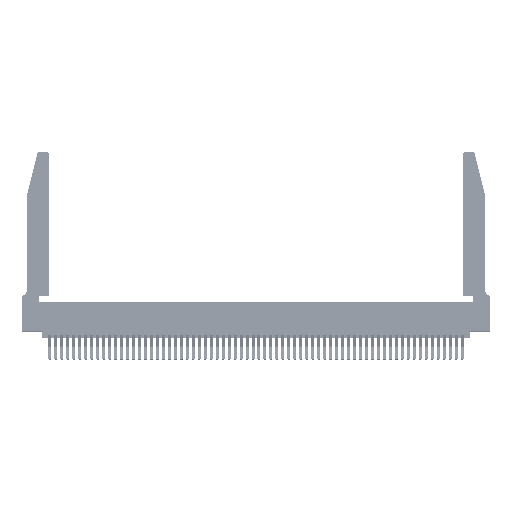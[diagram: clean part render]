
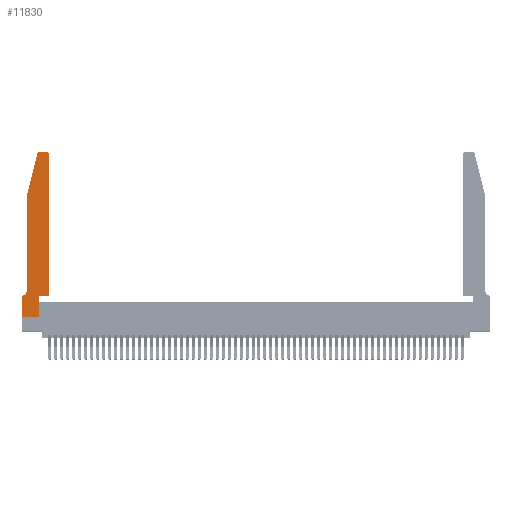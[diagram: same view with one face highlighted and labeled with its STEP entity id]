
A CAD part, top view. The second image highlights one B-rep face of the part: STEP entity #11830.
In plain terms, the highlighted planar face has unit normal (0, 0, 1).
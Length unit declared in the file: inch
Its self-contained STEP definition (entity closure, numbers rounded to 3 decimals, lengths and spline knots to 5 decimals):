
#631 = DIRECTION ( 'NONE',  ( 0., 0., 1. ) ) ;
#991 = LINE ( 'NONE', #21678, #45772 ) ;
#1443 = CARTESIAN_POINT ( 'NONE',  ( 0.4505, 0.35, 0.37 ) ) ;
#1514 = DIRECTION ( 'NONE',  ( 1., 0., 0. ) ) ;
#3117 = ORIENTED_EDGE ( 'NONE', *, *, #33888, .T. ) ;
#3269 = LINE ( 'NONE', #51267, #35183 ) ;
#3454 = CARTESIAN_POINT ( 'NONE',  ( 0.0755, 2., 0.37 ) ) ;
#3655 = VERTEX_POINT ( 'NONE', #53787 ) ;
#4149 = DIRECTION ( 'NONE',  ( 0., 0., 1. ) ) ;
#4368 = VERTEX_POINT ( 'NONE', #55041 ) ;
#4823 = VERTEX_POINT ( 'NONE', #53492 ) ;
#5504 = LINE ( 'NONE', #21820, #50225 ) ;
#7481 = CARTESIAN_POINT ( 'NONE',  ( 0.0055, 0.42, 0.37 ) ) ;
#7832 = DIRECTION ( 'NONE',  ( 0., -1., 0. ) ) ;
#9919 = ORIENTED_EDGE ( 'NONE', *, *, #21206, .T. ) ;
#10072 = EDGE_CURVE ( 'NONE', #13642, #23403, #991, .T. ) ;
#10275 = CARTESIAN_POINT ( 'NONE',  ( 0., 0., 0.37 ) ) ;
#10385 = VERTEX_POINT ( 'NONE', #10572 ) ;
#10572 = CARTESIAN_POINT ( 'NONE',  ( 0.284, 2.75, 0.37 ) ) ;
#10621 = CIRCLE ( 'NONE', #30736, 0.03 ) ;
#11830 = ADVANCED_FACE ( 'NONE', ( #29596 ), #52591, .T. ) ;
#11868 = DIRECTION ( 'NONE',  ( -1., 0., 0. ) ) ;
#13106 = ORIENTED_EDGE ( 'NONE', *, *, #21779, .T. ) ;
#13225 = DIRECTION ( 'NONE',  ( -1., 0., 0. ) ) ;
#13642 = VERTEX_POINT ( 'NONE', #27111 ) ;
#15131 = ORIENTED_EDGE ( 'NONE', *, *, #39594, .T. ) ;
#15133 = EDGE_CURVE ( 'NONE', #37219, #13642, #16375, .T. ) ;
#15163 = AXIS2_PLACEMENT_3D ( 'NONE', #22401, #631, #31086 ) ;
#15586 = EDGE_CURVE ( 'NONE', #3655, #22832, #49420, .T. ) ;
#16375 = CIRCLE ( 'NONE', #28686, 0.07 ) ;
#16689 = CARTESIAN_POINT ( 'NONE',  ( 0.4505, 0.35, 0.37 ) ) ;
#17494 = DIRECTION ( 'NONE',  ( -1., 0., 0. ) ) ;
#17820 = CARTESIAN_POINT ( 'NONE',  ( 0.4205, 2.75, 0.37 ) ) ;
#18159 = AXIS2_PLACEMENT_3D ( 'NONE', #30188, #4149, #34513 ) ;
#18362 = CARTESIAN_POINT ( 'NONE',  ( 0.25487, 2.72718, 0.37 ) ) ;
#18867 = ORIENTED_EDGE ( 'NONE', *, *, #54204, .T. ) ;
#18880 = VERTEX_POINT ( 'NONE', #17820 ) ;
#20620 = ORIENTED_EDGE ( 'NONE', *, *, #54653, .T. ) ;
#21063 = DIRECTION ( 'NONE',  ( 0., 1., 0. ) ) ;
#21206 = EDGE_CURVE ( 'NONE', #29919, #3655, #3269, .T. ) ;
#21678 = CARTESIAN_POINT ( 'NONE',  ( 0.0755, 0.35, 0.37 ) ) ;
#21779 = EDGE_CURVE ( 'NONE', #4823, #37219, #29715, .T. ) ;
#21820 = CARTESIAN_POINT ( 'NONE',  ( 0.2605, 2.75, 0.37 ) ) ;
#22352 = DIRECTION ( 'NONE',  ( 0., 0., 1. ) ) ;
#22401 = CARTESIAN_POINT ( 'NONE',  ( 0., 0.35, 0.37 ) ) ;
#22832 = VERTEX_POINT ( 'NONE', #1443 ) ;
#23403 = VERTEX_POINT ( 'NONE', #35562 ) ;
#24073 = CIRCLE ( 'NONE', #18159, 0.03 ) ;
#24998 = VERTEX_POINT ( 'NONE', #18362 ) ;
#27111 = CARTESIAN_POINT ( 'NONE',  ( 0.0055, 0.35, 0.37 ) ) ;
#27394 = LINE ( 'NONE', #41451, #50333 ) ;
#27542 = ORIENTED_EDGE ( 'NONE', *, *, #10072, .T. ) ;
#28374 = VECTOR ( 'NONE', #7832, 39.37008 ) ;
#28686 = AXIS2_PLACEMENT_3D ( 'NONE', #7481, #37790, #11868 ) ;
#29538 = ORIENTED_EDGE ( 'NONE', *, *, #15133, .T. ) ;
#29596 = FACE_OUTER_BOUND ( 'NONE', #49045, .T. ) ;
#29715 = LINE ( 'NONE', #3454, #28374 ) ;
#29919 = VERTEX_POINT ( 'NONE', #52624 ) ;
#30188 = CARTESIAN_POINT ( 'NONE',  ( 0.4205, 2.72, 0.37 ) ) ;
#30736 = AXIS2_PLACEMENT_3D ( 'NONE', #48177, #22352, #52539 ) ;
#31086 = DIRECTION ( 'NONE',  ( 1., 0., 0. ) ) ;
#33638 = ORIENTED_EDGE ( 'NONE', *, *, #54966, .T. ) ;
#33888 = EDGE_CURVE ( 'NONE', #22832, #54137, #46486, .T. ) ;
#34084 = LINE ( 'NONE', #34825, #55682 ) ;
#34489 = CARTESIAN_POINT ( 'NONE',  ( 0.0755, 0.42, 0.37 ) ) ;
#34513 = DIRECTION ( 'NONE',  ( 1., 0., 0. ) ) ;
#34825 = CARTESIAN_POINT ( 'NONE',  ( 0., 0., 0.37 ) ) ;
#35183 = VECTOR ( 'NONE', #51450, 39.37008 ) ;
#35562 = CARTESIAN_POINT ( 'NONE',  ( 0., 0.35, 0.37 ) ) ;
#37219 = VERTEX_POINT ( 'NONE', #34489 ) ;
#37790 = DIRECTION ( 'NONE',  ( 0., 0., -1. ) ) ;
#39594 = EDGE_CURVE ( 'NONE', #10385, #24998, #10621, .T. ) ;
#39710 = ORIENTED_EDGE ( 'NONE', *, *, #52754, .T. ) ;
#39756 = VECTOR ( 'NONE', #53610, 39.37008 ) ;
#41451 = CARTESIAN_POINT ( 'NONE',  ( 0.0755, 2., 0.37 ) ) ;
#42634 = CARTESIAN_POINT ( 'NONE',  ( 0.4505, 2.72, 0.37 ) ) ;
#44205 = ORIENTED_EDGE ( 'NONE', *, *, #47703, .T. ) ;
#45118 = VECTOR ( 'NONE', #21063, 39.37008 ) ;
#45772 = VECTOR ( 'NONE', #17494, 39.37008 ) ;
#46486 = LINE ( 'NONE', #16689, #45118 ) ;
#47703 = EDGE_CURVE ( 'NONE', #18880, #10385, #5504, .T. ) ;
#48070 = VECTOR ( 'NONE', #1514, 39.37008 ) ;
#48177 = CARTESIAN_POINT ( 'NONE',  ( 0.284, 2.72, 0.37 ) ) ;
#49045 = EDGE_LOOP ( 'NONE', ( #44205, #15131, #20620, #13106, #29538, #27542, #39710, #33638, #9919, #53953, #3117, #18867 ) ) ;
#49420 = LINE ( 'NONE', #53632, #48070 ) ;
#50143 = DIRECTION ( 'NONE',  ( -0.239, -0.971, 0. ) ) ;
#50225 = VECTOR ( 'NONE', #13225, 39.37008 ) ;
#50333 = VECTOR ( 'NONE', #50143, 39.37008 ) ;
#51223 = LINE ( 'NONE', #10275, #39756 ) ;
#51267 = CARTESIAN_POINT ( 'NONE',  ( 0.2865, 0.35, 0.37 ) ) ;
#51450 = DIRECTION ( 'NONE',  ( 0., 1., 0. ) ) ;
#52203 = DIRECTION ( 'NONE',  ( 1., 0., 0. ) ) ;
#52539 = DIRECTION ( 'NONE',  ( 1., 0., 0. ) ) ;
#52591 = PLANE ( 'NONE',  #15163 ) ;
#52624 = CARTESIAN_POINT ( 'NONE',  ( 0.2865, 0., 0.37 ) ) ;
#52754 = EDGE_CURVE ( 'NONE', #23403, #4368, #51223, .T. ) ;
#53492 = CARTESIAN_POINT ( 'NONE',  ( 0.0755, 2., 0.37 ) ) ;
#53610 = DIRECTION ( 'NONE',  ( 0., -1., 0. ) ) ;
#53632 = CARTESIAN_POINT ( 'NONE',  ( 0.4505, 0.35, 0.37 ) ) ;
#53787 = CARTESIAN_POINT ( 'NONE',  ( 0.2865, 0.35, 0.37 ) ) ;
#53953 = ORIENTED_EDGE ( 'NONE', *, *, #15586, .T. ) ;
#54137 = VERTEX_POINT ( 'NONE', #42634 ) ;
#54204 = EDGE_CURVE ( 'NONE', #54137, #18880, #24073, .T. ) ;
#54653 = EDGE_CURVE ( 'NONE', #24998, #4823, #27394, .T. ) ;
#54966 = EDGE_CURVE ( 'NONE', #4368, #29919, #34084, .T. ) ;
#55041 = CARTESIAN_POINT ( 'NONE',  ( 0., 0., 0.37 ) ) ;
#55682 = VECTOR ( 'NONE', #52203, 39.37008 ) ;
